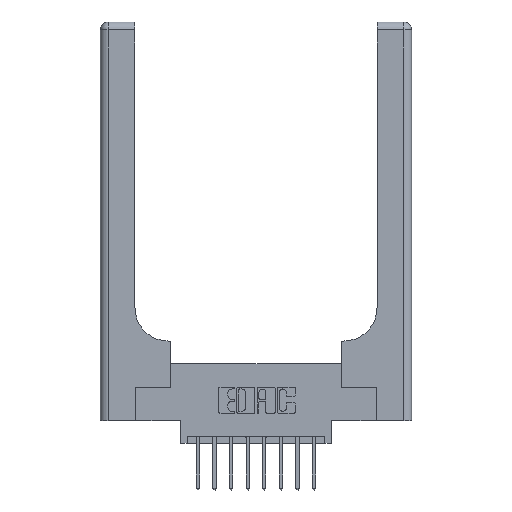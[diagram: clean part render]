
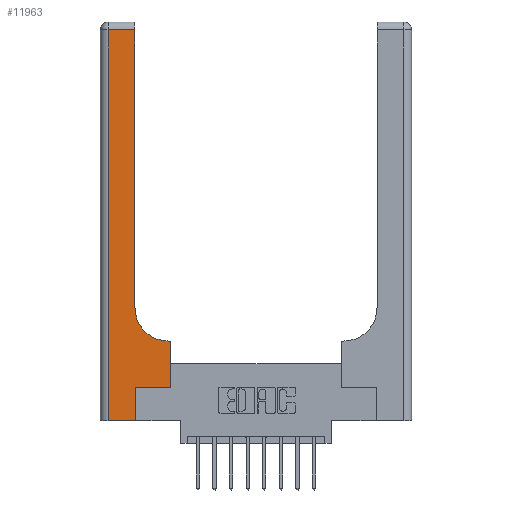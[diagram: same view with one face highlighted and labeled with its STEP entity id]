
A CAD part, top view. The second image highlights one B-rep face of the part: STEP entity #11963.
In plain terms, the highlighted planar face has unit normal (0, 0, 1).
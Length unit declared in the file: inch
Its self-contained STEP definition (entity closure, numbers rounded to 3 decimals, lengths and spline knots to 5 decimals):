
#15 = VERTEX_POINT ( 'NONE', #3772 ) ;
#67 = LINE ( 'NONE', #8268, #13873 ) ;
#553 = LINE ( 'NONE', #14002, #5532 ) ;
#591 = ORIENTED_EDGE ( 'NONE', *, *, #6469, .T. ) ;
#782 = LINE ( 'NONE', #3157, #5996 ) ;
#1126 = DIRECTION ( 'NONE',  ( 0., 0., -1. ) ) ;
#1373 = VERTEX_POINT ( 'NONE', #14659 ) ;
#1622 = CARTESIAN_POINT ( 'NONE',  ( 0.265, 0.25, 0.37 ) ) ;
#1655 = EDGE_CURVE ( 'NONE', #5364, #7621, #9803, .T. ) ;
#1711 = VECTOR ( 'NONE', #11164, 39.37008 ) ;
#1996 = VERTEX_POINT ( 'NONE', #10646 ) ;
#2235 = ORIENTED_EDGE ( 'NONE', *, *, #11734, .T. ) ;
#2923 = EDGE_CURVE ( 'NONE', #13391, #8092, #6999, .T. ) ;
#3063 = CARTESIAN_POINT ( 'NONE',  ( 0.265, 0.25, 0.37 ) ) ;
#3157 = CARTESIAN_POINT ( 'NONE',  ( 0.26, 0.6, 0.37 ) ) ;
#3553 = DIRECTION ( 'NONE',  ( 0., 1., 0. ) ) ;
#3594 = ORIENTED_EDGE ( 'NONE', *, *, #13845, .T. ) ;
#3719 = VECTOR ( 'NONE', #10670, 39.37008 ) ;
#3772 = CARTESIAN_POINT ( 'NONE',  ( 0.265, 0., 0.37 ) ) ;
#3812 = DIRECTION ( 'NONE',  ( 0., 1., 0. ) ) ;
#3887 = CARTESIAN_POINT ( 'NONE',  ( 0.265, 0., 0.37 ) ) ;
#4077 = LINE ( 'NONE', #1622, #10748 ) ;
#4709 = LINE ( 'NONE', #13459, #1711 ) ;
#5364 = VERTEX_POINT ( 'NONE', #5862 ) ;
#5532 = VECTOR ( 'NONE', #15347, 39.37008 ) ;
#5862 = CARTESIAN_POINT ( 'NONE',  ( 0.51, 0.6, 0.37 ) ) ;
#5996 = VECTOR ( 'NONE', #7078, 39.37008 ) ;
#6469 = EDGE_CURVE ( 'NONE', #7621, #10897, #4709, .T. ) ;
#6895 = CARTESIAN_POINT ( 'NONE',  ( 0., 0., 0.37 ) ) ;
#6988 = CARTESIAN_POINT ( 'NONE',  ( 0.26, 0.85, 0.37 ) ) ;
#6999 = LINE ( 'NONE', #11889, #13680 ) ;
#7063 = DIRECTION ( 'NONE',  ( 1., 0., 0. ) ) ;
#7078 = DIRECTION ( 'NONE',  ( -1., 0., 0. ) ) ;
#7557 = EDGE_CURVE ( 'NONE', #10897, #1373, #553, .T. ) ;
#7621 = VERTEX_POINT ( 'NONE', #6988 ) ;
#7665 = ORIENTED_EDGE ( 'NONE', *, *, #13498, .T. ) ;
#7684 = DIRECTION ( 'NONE',  ( 1., 0., 0. ) ) ;
#7745 = VECTOR ( 'NONE', #3812, 39.37008 ) ;
#8092 = VERTEX_POINT ( 'NONE', #9111 ) ;
#8268 = CARTESIAN_POINT ( 'NONE',  ( 0.06, 3., 0.37 ) ) ;
#9111 = CARTESIAN_POINT ( 'NONE',  ( 0.528, 0.6, 0.37 ) ) ;
#9263 = VERTEX_POINT ( 'NONE', #3063 ) ;
#9426 = ORIENTED_EDGE ( 'NONE', *, *, #11416, .T. ) ;
#9554 = PLANE ( 'NONE',  #13755 ) ;
#9724 = ORIENTED_EDGE ( 'NONE', *, *, #11112, .T. ) ;
#9772 = LINE ( 'NONE', #3887, #7745 ) ;
#9803 = CIRCLE ( 'NONE', #14324, 0.25 ) ;
#10646 = CARTESIAN_POINT ( 'NONE',  ( 0.06, 0., 0.37 ) ) ;
#10670 = DIRECTION ( 'NONE',  ( 1., 0., 0. ) ) ;
#10688 = DIRECTION ( 'NONE',  ( 0., -1., 0. ) ) ;
#10746 = LINE ( 'NONE', #6895, #3719 ) ;
#10748 = VECTOR ( 'NONE', #7684, 39.37008 ) ;
#10760 = CARTESIAN_POINT ( 'NONE',  ( 0.51, 0.85, 0.37 ) ) ;
#10897 = VERTEX_POINT ( 'NONE', #12741 ) ;
#11112 = EDGE_CURVE ( 'NONE', #1373, #1996, #67, .T. ) ;
#11164 = DIRECTION ( 'NONE',  ( 0., 1., 0. ) ) ;
#11416 = EDGE_CURVE ( 'NONE', #1996, #15, #10746, .T. ) ;
#11734 = EDGE_CURVE ( 'NONE', #9263, #13391, #4077, .T. ) ;
#11751 = FACE_OUTER_BOUND ( 'NONE', #13243, .T. ) ;
#11889 = CARTESIAN_POINT ( 'NONE',  ( 0.528, 0.25, 0.37 ) ) ;
#11920 = CARTESIAN_POINT ( 'NONE',  ( 0., 3., 0.37 ) ) ;
#11963 = ADVANCED_FACE ( 'NONE', ( #11751 ), #9554, .F. ) ;
#12145 = ORIENTED_EDGE ( 'NONE', *, *, #1655, .T. ) ;
#12741 = CARTESIAN_POINT ( 'NONE',  ( 0.26, 2.94, 0.37 ) ) ;
#12946 = ORIENTED_EDGE ( 'NONE', *, *, #2923, .T. ) ;
#13094 = CARTESIAN_POINT ( 'NONE',  ( 0.528, 0.25, 0.37 ) ) ;
#13136 = ORIENTED_EDGE ( 'NONE', *, *, #7557, .T. ) ;
#13243 = EDGE_LOOP ( 'NONE', ( #591, #13136, #9724, #9426, #7665, #2235, #12946, #3594, #12145 ) ) ;
#13391 = VERTEX_POINT ( 'NONE', #13094 ) ;
#13459 = CARTESIAN_POINT ( 'NONE',  ( 0.26, 3., 0.37 ) ) ;
#13498 = EDGE_CURVE ( 'NONE', #15, #9263, #9772, .T. ) ;
#13680 = VECTOR ( 'NONE', #3553, 39.37008 ) ;
#13755 = AXIS2_PLACEMENT_3D ( 'NONE', #11920, #1126, #14127 ) ;
#13845 = EDGE_CURVE ( 'NONE', #8092, #5364, #782, .T. ) ;
#13873 = VECTOR ( 'NONE', #10688, 39.37008 ) ;
#14002 = CARTESIAN_POINT ( 'NONE',  ( 0., 2.94, 0.37 ) ) ;
#14127 = DIRECTION ( 'NONE',  ( -1., 0., 0. ) ) ;
#14230 = DIRECTION ( 'NONE',  ( 0., 0., -1. ) ) ;
#14324 = AXIS2_PLACEMENT_3D ( 'NONE', #10760, #14230, #7063 ) ;
#14659 = CARTESIAN_POINT ( 'NONE',  ( 0.06, 2.94, 0.37 ) ) ;
#15347 = DIRECTION ( 'NONE',  ( -1., 0., 0. ) ) ;
